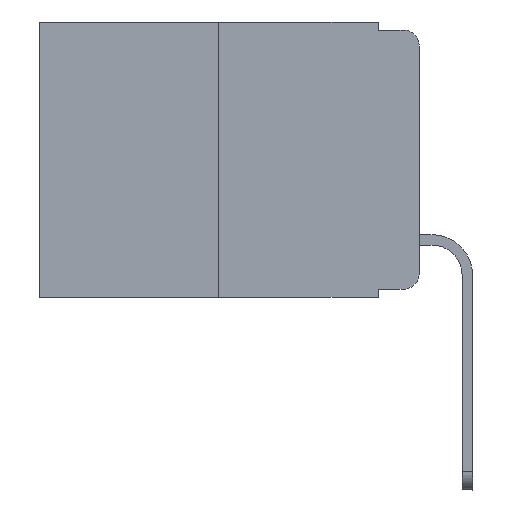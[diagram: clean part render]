
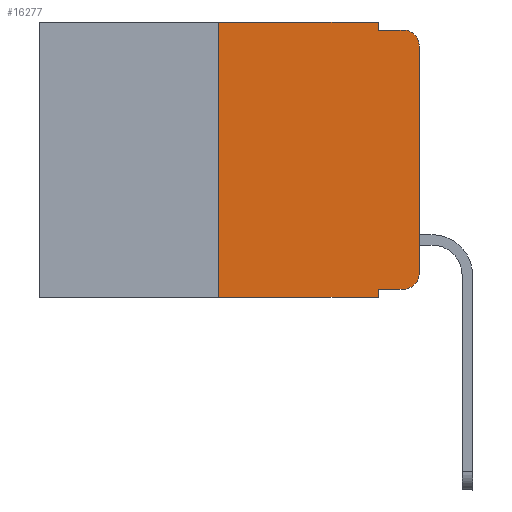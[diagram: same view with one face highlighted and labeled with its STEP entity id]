
A CAD part, left-side view. The second image highlights one B-rep face of the part: STEP entity #16277.
In plain terms, the highlighted planar face has unit normal (-1, 0, 0).
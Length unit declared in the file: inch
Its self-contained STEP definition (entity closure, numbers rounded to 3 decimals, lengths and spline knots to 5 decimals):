
#3 = CARTESIAN_POINT ( 'NONE',  ( 0., 0.051, 0. ) ) ;
#414 = CARTESIAN_POINT ( 'NONE',  ( 0., 0.25, -0.343 ) ) ;
#453 = VECTOR ( 'NONE', #1392, 39.37008 ) ;
#504 = EDGE_CURVE ( 'NONE', #5151, #5641, #3926, .T. ) ;
#631 = ORIENTED_EDGE ( 'NONE', *, *, #11629, .T. ) ;
#653 = VECTOR ( 'NONE', #6863, 39.37008 ) ;
#693 = DIRECTION ( 'NONE',  ( 0., 0., 1. ) ) ;
#705 = DIRECTION ( 'NONE',  ( 0., 0., -1. ) ) ;
#786 = CARTESIAN_POINT ( 'NONE',  ( 0., 0.473, 0. ) ) ;
#1392 = DIRECTION ( 'NONE',  ( 0., 0., -1. ) ) ;
#1585 = CARTESIAN_POINT ( 'NONE',  ( 0., 0.25, 0. ) ) ;
#1763 = DIRECTION ( 'NONE',  ( 0., 0., -1. ) ) ;
#1903 = CARTESIAN_POINT ( 'NONE',  ( 0., 0.051, 0. ) ) ;
#1919 = CARTESIAN_POINT ( 'NONE',  ( 0., 0., -0.313 ) ) ;
#2023 = DIRECTION ( 'NONE',  ( 0., -1., 0. ) ) ;
#2326 = CARTESIAN_POINT ( 'NONE',  ( 0., 0., 0. ) ) ;
#2405 = ORIENTED_EDGE ( 'NONE', *, *, #6586, .F. ) ;
#2747 = DIRECTION ( 'NONE',  ( 0., 0., -1. ) ) ;
#2981 = EDGE_CURVE ( 'NONE', #5641, #14925, #3540, .T. ) ;
#3076 = CARTESIAN_POINT ( 'NONE',  ( 0., 0.473, 0. ) ) ;
#3222 = VERTEX_POINT ( 'NONE', #3786 ) ;
#3540 = LINE ( 'NONE', #2326, #10196 ) ;
#3560 = CARTESIAN_POINT ( 'NONE',  ( 0., 0.051, -0.333 ) ) ;
#3786 = CARTESIAN_POINT ( 'NONE',  ( 0., 0.051, -0.01 ) ) ;
#3926 = CIRCLE ( 'NONE', #8893, 0.02 ) ;
#4017 = DIRECTION ( 'NONE',  ( 0., -1., 0. ) ) ;
#4164 = VECTOR ( 'NONE', #6815, 39.37008 ) ;
#4270 = ORIENTED_EDGE ( 'NONE', *, *, #4570, .F. ) ;
#4570 = EDGE_CURVE ( 'NONE', #8467, #14624, #5290, .T. ) ;
#4620 = CARTESIAN_POINT ( 'NONE',  ( 0., 0.473, -0.343 ) ) ;
#4748 = CIRCLE ( 'NONE', #8312, 0.02 ) ;
#5087 = VECTOR ( 'NONE', #2023, 39.37008 ) ;
#5151 = VERTEX_POINT ( 'NONE', #15083 ) ;
#5290 = LINE ( 'NONE', #6748, #453 ) ;
#5442 = LINE ( 'NONE', #3, #4164 ) ;
#5554 = CARTESIAN_POINT ( 'NONE',  ( 0., 0.02, -0.01 ) ) ;
#5641 = VERTEX_POINT ( 'NONE', #1919 ) ;
#6371 = ORIENTED_EDGE ( 'NONE', *, *, #14673, .F. ) ;
#6445 = CARTESIAN_POINT ( 'NONE',  ( 0., 0.051, -0.01 ) ) ;
#6586 = EDGE_CURVE ( 'NONE', #7903, #14008, #10578, .T. ) ;
#6648 = ORIENTED_EDGE ( 'NONE', *, *, #9617, .F. ) ;
#6689 = LINE ( 'NONE', #14375, #7334 ) ;
#6729 = EDGE_CURVE ( 'NONE', #7903, #14624, #11164, .T. ) ;
#6748 = CARTESIAN_POINT ( 'NONE',  ( 0., 0.051, 0. ) ) ;
#6815 = DIRECTION ( 'NONE',  ( 0., 0., -1. ) ) ;
#6863 = DIRECTION ( 'NONE',  ( 0., 0., 1. ) ) ;
#7334 = VECTOR ( 'NONE', #7815, 39.37008 ) ;
#7815 = DIRECTION ( 'NONE',  ( 0., -1., 0. ) ) ;
#7903 = VERTEX_POINT ( 'NONE', #414 ) ;
#8008 = DIRECTION ( 'NONE',  ( -1., 0., 0. ) ) ;
#8130 = VERTEX_POINT ( 'NONE', #5554 ) ;
#8312 = AXIS2_PLACEMENT_3D ( 'NONE', #16245, #13587, #1763 ) ;
#8467 = VERTEX_POINT ( 'NONE', #3560 ) ;
#8474 = FACE_OUTER_BOUND ( 'NONE', #10766, .T. ) ;
#8893 = AXIS2_PLACEMENT_3D ( 'NONE', #9303, #8008, #2747 ) ;
#9303 = CARTESIAN_POINT ( 'NONE',  ( 0., 0.02, -0.313 ) ) ;
#9429 = VECTOR ( 'NONE', #12219, 39.37008 ) ;
#9537 = LINE ( 'NONE', #3076, #9429 ) ;
#9617 = EDGE_CURVE ( 'NONE', #14008, #13641, #9537, .T. ) ;
#9671 = ORIENTED_EDGE ( 'NONE', *, *, #2981, .T. ) ;
#10196 = VECTOR ( 'NONE', #693, 39.37008 ) ;
#10578 = LINE ( 'NONE', #1585, #653 ) ;
#10766 = EDGE_LOOP ( 'NONE', ( #9671, #16841, #12652, #6371, #6648, #2405, #13121, #4270, #631, #14536 ) ) ;
#11143 = PLANE ( 'NONE',  #12733 ) ;
#11164 = LINE ( 'NONE', #4620, #5087 ) ;
#11629 = EDGE_CURVE ( 'NONE', #8467, #5151, #6689, .T. ) ;
#11928 = VECTOR ( 'NONE', #4017, 39.37008 ) ;
#12219 = DIRECTION ( 'NONE',  ( 0., -1., 0. ) ) ;
#12399 = CARTESIAN_POINT ( 'NONE',  ( 0., 0.25, 0. ) ) ;
#12652 = ORIENTED_EDGE ( 'NONE', *, *, #16797, .F. ) ;
#12733 = AXIS2_PLACEMENT_3D ( 'NONE', #786, #13903, #705 ) ;
#13121 = ORIENTED_EDGE ( 'NONE', *, *, #6729, .T. ) ;
#13587 = DIRECTION ( 'NONE',  ( -1., 0., 0. ) ) ;
#13641 = VERTEX_POINT ( 'NONE', #1903 ) ;
#13707 = CARTESIAN_POINT ( 'NONE',  ( 0., 0., -0.03 ) ) ;
#13863 = LINE ( 'NONE', #6445, #11928 ) ;
#13903 = DIRECTION ( 'NONE',  ( 1., 0., 0. ) ) ;
#14008 = VERTEX_POINT ( 'NONE', #12399 ) ;
#14375 = CARTESIAN_POINT ( 'NONE',  ( 0., 0.051, -0.333 ) ) ;
#14536 = ORIENTED_EDGE ( 'NONE', *, *, #504, .T. ) ;
#14624 = VERTEX_POINT ( 'NONE', #16639 ) ;
#14673 = EDGE_CURVE ( 'NONE', #13641, #3222, #5442, .T. ) ;
#14925 = VERTEX_POINT ( 'NONE', #13707 ) ;
#15083 = CARTESIAN_POINT ( 'NONE',  ( 0., 0.02, -0.333 ) ) ;
#15743 = EDGE_CURVE ( 'NONE', #14925, #8130, #4748, .T. ) ;
#16245 = CARTESIAN_POINT ( 'NONE',  ( 0., 0.02, -0.03 ) ) ;
#16277 = ADVANCED_FACE ( 'NONE', ( #8474 ), #11143, .F. ) ;
#16639 = CARTESIAN_POINT ( 'NONE',  ( 0., 0.051, -0.343 ) ) ;
#16797 = EDGE_CURVE ( 'NONE', #3222, #8130, #13863, .T. ) ;
#16841 = ORIENTED_EDGE ( 'NONE', *, *, #15743, .T. ) ;
